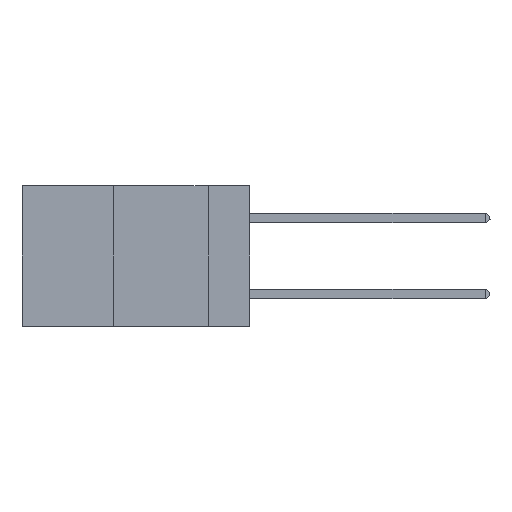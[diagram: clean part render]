
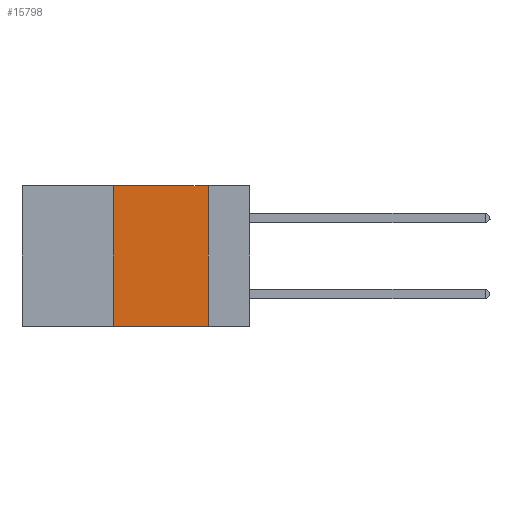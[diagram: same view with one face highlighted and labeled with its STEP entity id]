
A CAD part, left-side view. The second image highlights one B-rep face of the part: STEP entity #15798.
In plain terms, the highlighted planar face has unit normal (-1, 0, 0).
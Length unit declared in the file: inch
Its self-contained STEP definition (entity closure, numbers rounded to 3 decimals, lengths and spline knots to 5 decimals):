
#950 = DIRECTION ( 'NONE',  ( 0., 0., -1. ) ) ;
#1109 = EDGE_CURVE ( 'NONE', #4352, #1363, #4587, .T. ) ;
#1363 = VERTEX_POINT ( 'NONE', #12773 ) ;
#1484 = VECTOR ( 'NONE', #12770, 39.37008 ) ;
#1691 = CARTESIAN_POINT ( 'NONE',  ( 0., 0.11, 0. ) ) ;
#1832 = EDGE_CURVE ( 'NONE', #4352, #15554, #17334, .T. ) ;
#2451 = CARTESIAN_POINT ( 'NONE',  ( 0., 0.6, 0. ) ) ;
#2707 = CARTESIAN_POINT ( 'NONE',  ( 0., 0.11, 0. ) ) ;
#2964 = EDGE_CURVE ( 'NONE', #15554, #3021, #16855, .T. ) ;
#3000 = EDGE_LOOP ( 'NONE', ( #5202, #17161, #14359, #8499 ) ) ;
#3021 = VERTEX_POINT ( 'NONE', #1691 ) ;
#3963 = CARTESIAN_POINT ( 'NONE',  ( 0., 0.6, 0. ) ) ;
#4159 = CARTESIAN_POINT ( 'NONE',  ( 0., 0.36, 0. ) ) ;
#4222 = VECTOR ( 'NONE', #9698, 39.37008 ) ;
#4352 = VERTEX_POINT ( 'NONE', #5300 ) ;
#4587 = LINE ( 'NONE', #13066, #7377 ) ;
#5202 = ORIENTED_EDGE ( 'NONE', *, *, #5286, .F. ) ;
#5286 = EDGE_CURVE ( 'NONE', #3021, #1363, #12954, .T. ) ;
#5300 = CARTESIAN_POINT ( 'NONE',  ( 0., 0.36, -0.37 ) ) ;
#7377 = VECTOR ( 'NONE', #10520, 39.37008 ) ;
#7811 = DIRECTION ( 'NONE',  ( 1., 0., 0. ) ) ;
#8178 = FACE_OUTER_BOUND ( 'NONE', #3000, .T. ) ;
#8302 = CARTESIAN_POINT ( 'NONE',  ( 0., 0.36, 0. ) ) ;
#8499 = ORIENTED_EDGE ( 'NONE', *, *, #1109, .T. ) ;
#9201 = VECTOR ( 'NONE', #15631, 39.37008 ) ;
#9698 = DIRECTION ( 'NONE',  ( 0., -1., 0. ) ) ;
#10520 = DIRECTION ( 'NONE',  ( 0., -1., 0. ) ) ;
#12770 = DIRECTION ( 'NONE',  ( 0., 0., -1. ) ) ;
#12773 = CARTESIAN_POINT ( 'NONE',  ( 0., 0.11, -0.37 ) ) ;
#12954 = LINE ( 'NONE', #2707, #1484 ) ;
#13066 = CARTESIAN_POINT ( 'NONE',  ( 0., 0.6, -0.37 ) ) ;
#14359 = ORIENTED_EDGE ( 'NONE', *, *, #1832, .F. ) ;
#14705 = AXIS2_PLACEMENT_3D ( 'NONE', #2451, #7811, #950 ) ;
#15554 = VERTEX_POINT ( 'NONE', #8302 ) ;
#15631 = DIRECTION ( 'NONE',  ( 0., 0., 1. ) ) ;
#15798 = ADVANCED_FACE ( 'NONE', ( #8178 ), #16472, .F. ) ;
#16472 = PLANE ( 'NONE',  #14705 ) ;
#16855 = LINE ( 'NONE', #3963, #4222 ) ;
#17161 = ORIENTED_EDGE ( 'NONE', *, *, #2964, .F. ) ;
#17334 = LINE ( 'NONE', #4159, #9201 ) ;
